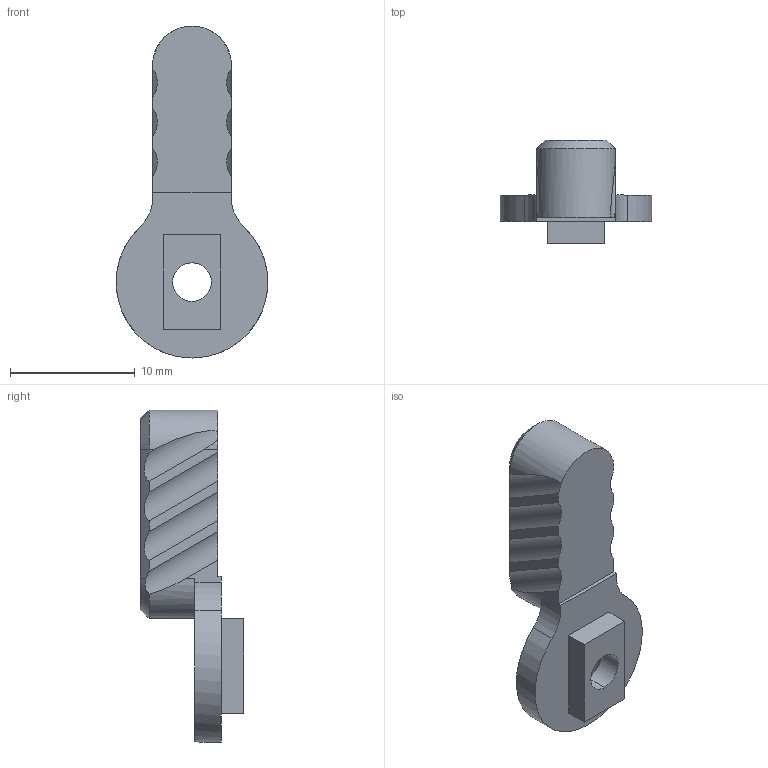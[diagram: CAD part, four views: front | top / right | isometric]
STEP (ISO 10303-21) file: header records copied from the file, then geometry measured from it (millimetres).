
FILE_DESCRIPTION (( 'STEP AP214' ), '1' );
FILE_NAME ('Lever_Standard.step', '2015-07-11T17:33:21', ( 'WarFairy' ), ( '' ), 'SwSTEP 2.0', 'SolidWorks 2015', '' );
FILE_SCHEMA (( 'AUTOMOTIVE_DESIGN' ));
Length unit declared in the file: millimetre
Products named in the file (1): Lever_Standard
Bounding box: 12.17 x 8.29 x 26.63 mm (x, y, z)
Volume: 798.9 mm3; surface area: 780.6 mm2
Topology: 1 solids, 1 shells, 60 faces, 163 edges, 104 vertices
Faces by surface type: plane 27, cylinder 21, cone 8, torus 4
Entity records: 1950 total; most frequent: CARTESIAN_POINT 451, ORIENTED_EDGE 320, DIRECTION 296, EDGE_CURVE 160, VERTEX_POINT 104, AXIS2_PLACEMENT_3D 103, VECTOR 90, LINE 90
